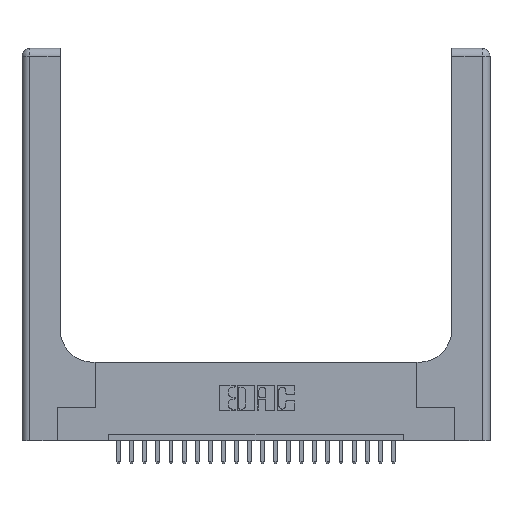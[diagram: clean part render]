
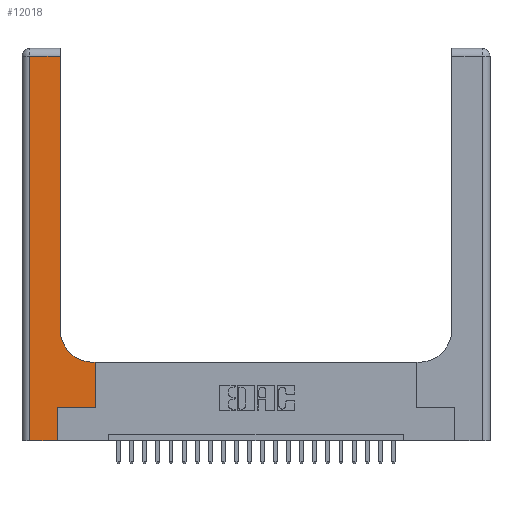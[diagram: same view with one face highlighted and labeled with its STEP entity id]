
A CAD part, top view. The second image highlights one B-rep face of the part: STEP entity #12018.
In plain terms, the highlighted planar face has unit normal (0, 0, 1).
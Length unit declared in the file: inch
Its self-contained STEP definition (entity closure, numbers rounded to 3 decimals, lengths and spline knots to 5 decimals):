
#378 = CARTESIAN_POINT ( 'NONE',  ( 0., 2.94, 0.37 ) ) ;
#471 = CARTESIAN_POINT ( 'NONE',  ( 0., 3., 0.37 ) ) ;
#635 = VECTOR ( 'NONE', #3000, 39.37008 ) ;
#1383 = VECTOR ( 'NONE', #3482, 39.37008 ) ;
#1577 = LINE ( 'NONE', #378, #22008 ) ;
#2207 = PLANE ( 'NONE',  #22945 ) ;
#2382 = LINE ( 'NONE', #22377, #5036 ) ;
#2698 = CARTESIAN_POINT ( 'NONE',  ( 0.269, 0., 0.37 ) ) ;
#3000 = DIRECTION ( 'NONE',  ( 0., -1., 0. ) ) ;
#3039 = VECTOR ( 'NONE', #13815, 39.37008 ) ;
#3206 = AXIS2_PLACEMENT_3D ( 'NONE', #5521, #22618, #11237 ) ;
#3442 = LINE ( 'NONE', #13266, #7875 ) ;
#3482 = DIRECTION ( 'NONE',  ( -1., 0., 0. ) ) ;
#3559 = ORIENTED_EDGE ( 'NONE', *, *, #13383, .T. ) ;
#4028 = ORIENTED_EDGE ( 'NONE', *, *, #11018, .T. ) ;
#4638 = DIRECTION ( 'NONE',  ( -1., 0., 0. ) ) ;
#4707 = ORIENTED_EDGE ( 'NONE', *, *, #8125, .T. ) ;
#5036 = VECTOR ( 'NONE', #22064, 39.37008 ) ;
#5521 = CARTESIAN_POINT ( 'NONE',  ( 0.5415, 0.85, 0.37 ) ) ;
#6372 = LINE ( 'NONE', #14902, #1383 ) ;
#6722 = EDGE_CURVE ( 'NONE', #6784, #14063, #1577, .T. ) ;
#6784 = VERTEX_POINT ( 'NONE', #19633 ) ;
#7001 = DIRECTION ( 'NONE',  ( 1., 0., 0. ) ) ;
#7613 = ORIENTED_EDGE ( 'NONE', *, *, #6722, .T. ) ;
#7661 = ORIENTED_EDGE ( 'NONE', *, *, #18673, .T. ) ;
#7731 = DIRECTION ( 'NONE',  ( -1., 0., 0. ) ) ;
#7875 = VECTOR ( 'NONE', #18975, 39.37008 ) ;
#8125 = EDGE_CURVE ( 'NONE', #8950, #20507, #10059, .T. ) ;
#8160 = VERTEX_POINT ( 'NONE', #15202 ) ;
#8465 = VERTEX_POINT ( 'NONE', #19849 ) ;
#8714 = CARTESIAN_POINT ( 'NONE',  ( 0., 0., 0.37 ) ) ;
#8950 = VERTEX_POINT ( 'NONE', #10595 ) ;
#8966 = EDGE_CURVE ( 'NONE', #20507, #6784, #17741, .T. ) ;
#10059 = CIRCLE ( 'NONE', #3206, 0.25 ) ;
#10107 = VERTEX_POINT ( 'NONE', #13338 ) ;
#10595 = CARTESIAN_POINT ( 'NONE',  ( 0.5415, 0.6, 0.37 ) ) ;
#10688 = EDGE_CURVE ( 'NONE', #10841, #8950, #6372, .T. ) ;
#10841 = VERTEX_POINT ( 'NONE', #13570 ) ;
#11018 = EDGE_CURVE ( 'NONE', #15497, #8465, #3442, .T. ) ;
#11237 = DIRECTION ( 'NONE',  ( 1., 0., 0. ) ) ;
#11444 = CARTESIAN_POINT ( 'NONE',  ( 0.2915, 3., 0.37 ) ) ;
#12018 = ADVANCED_FACE ( 'NONE', ( #18503 ), #2207, .F. ) ;
#12878 = CARTESIAN_POINT ( 'NONE',  ( 0.2915, 0.85, 0.37 ) ) ;
#13266 = CARTESIAN_POINT ( 'NONE',  ( 0.269, 0., 0.37 ) ) ;
#13338 = CARTESIAN_POINT ( 'NONE',  ( 0.5585, 0.25, 0.37 ) ) ;
#13383 = EDGE_CURVE ( 'NONE', #10107, #10841, #19303, .T. ) ;
#13570 = CARTESIAN_POINT ( 'NONE',  ( 0.5585, 0.6, 0.37 ) ) ;
#13815 = DIRECTION ( 'NONE',  ( 0., 1., 0. ) ) ;
#14063 = VERTEX_POINT ( 'NONE', #21532 ) ;
#14331 = EDGE_CURVE ( 'NONE', #8465, #10107, #2382, .T. ) ;
#14333 = CARTESIAN_POINT ( 'NONE',  ( 0.06, 3., 0.37 ) ) ;
#14902 = CARTESIAN_POINT ( 'NONE',  ( 0.2915, 0.6, 0.37 ) ) ;
#14908 = ORIENTED_EDGE ( 'NONE', *, *, #10688, .T. ) ;
#15202 = CARTESIAN_POINT ( 'NONE',  ( 0.06, 0., 0.37 ) ) ;
#15497 = VERTEX_POINT ( 'NONE', #2698 ) ;
#15617 = VECTOR ( 'NONE', #7001, 39.37008 ) ;
#15898 = LINE ( 'NONE', #8714, #15617 ) ;
#15938 = EDGE_LOOP ( 'NONE', ( #23711, #7613, #21862, #7661, #4028, #17712, #3559, #14908, #4707 ) ) ;
#16234 = EDGE_CURVE ( 'NONE', #14063, #8160, #18379, .T. ) ;
#17192 = CARTESIAN_POINT ( 'NONE',  ( 0.5585, 0.25, 0.37 ) ) ;
#17712 = ORIENTED_EDGE ( 'NONE', *, *, #14331, .T. ) ;
#17741 = LINE ( 'NONE', #11444, #22203 ) ;
#18379 = LINE ( 'NONE', #14333, #635 ) ;
#18503 = FACE_OUTER_BOUND ( 'NONE', #15938, .T. ) ;
#18673 = EDGE_CURVE ( 'NONE', #8160, #15497, #15898, .T. ) ;
#18975 = DIRECTION ( 'NONE',  ( 0., 1., 0. ) ) ;
#19303 = LINE ( 'NONE', #17192, #3039 ) ;
#19633 = CARTESIAN_POINT ( 'NONE',  ( 0.2915, 2.94, 0.37 ) ) ;
#19849 = CARTESIAN_POINT ( 'NONE',  ( 0.269, 0.25, 0.37 ) ) ;
#20507 = VERTEX_POINT ( 'NONE', #12878 ) ;
#21532 = CARTESIAN_POINT ( 'NONE',  ( 0.06, 2.94, 0.37 ) ) ;
#21862 = ORIENTED_EDGE ( 'NONE', *, *, #16234, .T. ) ;
#22008 = VECTOR ( 'NONE', #4638, 39.37008 ) ;
#22064 = DIRECTION ( 'NONE',  ( 1., 0., 0. ) ) ;
#22203 = VECTOR ( 'NONE', #22389, 39.37008 ) ;
#22377 = CARTESIAN_POINT ( 'NONE',  ( 0.269, 0.25, 0.37 ) ) ;
#22389 = DIRECTION ( 'NONE',  ( 0., 1., 0. ) ) ;
#22618 = DIRECTION ( 'NONE',  ( 0., 0., -1. ) ) ;
#22848 = DIRECTION ( 'NONE',  ( 0., 0., -1. ) ) ;
#22945 = AXIS2_PLACEMENT_3D ( 'NONE', #471, #22848, #7731 ) ;
#23711 = ORIENTED_EDGE ( 'NONE', *, *, #8966, .T. ) ;
